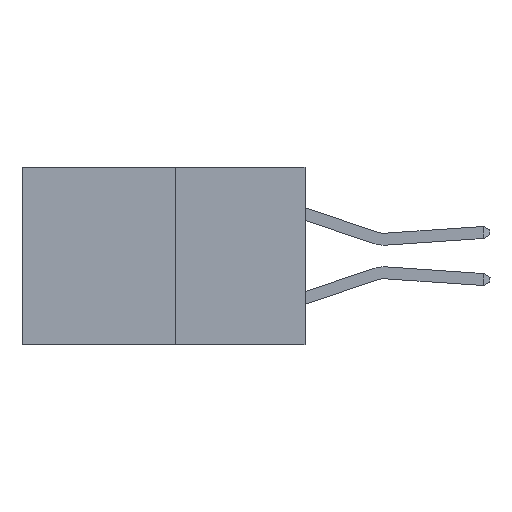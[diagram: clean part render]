
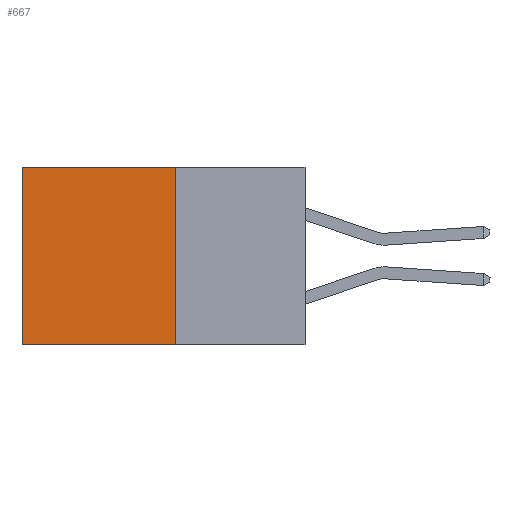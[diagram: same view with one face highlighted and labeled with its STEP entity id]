
A CAD part, left-side view. The second image highlights one B-rep face of the part: STEP entity #667.
In plain terms, the highlighted planar face has unit normal (-1, 0, 0).
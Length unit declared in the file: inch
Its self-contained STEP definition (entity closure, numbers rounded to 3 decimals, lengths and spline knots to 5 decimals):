
#667 = ADVANCED_FACE ( 'NONE', ( #1356 ), #22601, .F. ) ;
#778 = ORIENTED_EDGE ( 'NONE', *, *, #12205, .T. ) ;
#969 = CARTESIAN_POINT ( 'NONE',  ( 0.277, 0.27, -0.37 ) ) ;
#1356 = FACE_OUTER_BOUND ( 'NONE', #3260, .T. ) ;
#1427 = EDGE_CURVE ( 'NONE', #15576, #5607, #23389, .T. ) ;
#2685 = LINE ( 'NONE', #4295, #11202 ) ;
#3260 = EDGE_LOOP ( 'NONE', ( #8750, #9344, #19711, #778 ) ) ;
#3858 = CARTESIAN_POINT ( 'NONE',  ( 0.277, 0.27, 0. ) ) ;
#4284 = CARTESIAN_POINT ( 'NONE',  ( 0.277, 0.59, -0.37 ) ) ;
#4295 = CARTESIAN_POINT ( 'NONE',  ( 0.277, 0.59, -0.37 ) ) ;
#4622 = DIRECTION ( 'NONE',  ( 0., 1., 0. ) ) ;
#4705 = DIRECTION ( 'NONE',  ( 0., 0., -1. ) ) ;
#4827 = CARTESIAN_POINT ( 'NONE',  ( 0.277, 0.27, -0.37 ) ) ;
#5607 = VERTEX_POINT ( 'NONE', #21751 ) ;
#6101 = EDGE_CURVE ( 'NONE', #16688, #24304, #2685, .T. ) ;
#6717 = DIRECTION ( 'NONE',  ( 0., 0., -1. ) ) ;
#7148 = EDGE_CURVE ( 'NONE', #5607, #24304, #9970, .T. ) ;
#8750 = ORIENTED_EDGE ( 'NONE', *, *, #6101, .T. ) ;
#9344 = ORIENTED_EDGE ( 'NONE', *, *, #7148, .F. ) ;
#9970 = LINE ( 'NONE', #4827, #17946 ) ;
#11202 = VECTOR ( 'NONE', #12395, 39.37008 ) ;
#12205 = EDGE_CURVE ( 'NONE', #15576, #16688, #22592, .T. ) ;
#12395 = DIRECTION ( 'NONE',  ( 0., 0., -1. ) ) ;
#12539 = AXIS2_PLACEMENT_3D ( 'NONE', #22577, #14520, #4705 ) ;
#12876 = VECTOR ( 'NONE', #19155, 39.37008 ) ;
#14520 = DIRECTION ( 'NONE',  ( 1., 0., 0. ) ) ;
#15576 = VERTEX_POINT ( 'NONE', #3858 ) ;
#16688 = VERTEX_POINT ( 'NONE', #20194 ) ;
#17946 = VECTOR ( 'NONE', #4622, 39.37008 ) ;
#18499 = VECTOR ( 'NONE', #6717, 39.37008 ) ;
#19155 = DIRECTION ( 'NONE',  ( 0., 1., 0. ) ) ;
#19711 = ORIENTED_EDGE ( 'NONE', *, *, #1427, .F. ) ;
#20194 = CARTESIAN_POINT ( 'NONE',  ( 0.277, 0.59, 0. ) ) ;
#20952 = CARTESIAN_POINT ( 'NONE',  ( 0.277, 0.27, 0. ) ) ;
#21751 = CARTESIAN_POINT ( 'NONE',  ( 0.277, 0.27, -0.37 ) ) ;
#22577 = CARTESIAN_POINT ( 'NONE',  ( 0.277, 0.27, -0.37 ) ) ;
#22592 = LINE ( 'NONE', #20952, #12876 ) ;
#22601 = PLANE ( 'NONE',  #12539 ) ;
#23389 = LINE ( 'NONE', #969, #18499 ) ;
#24304 = VERTEX_POINT ( 'NONE', #4284 ) ;
